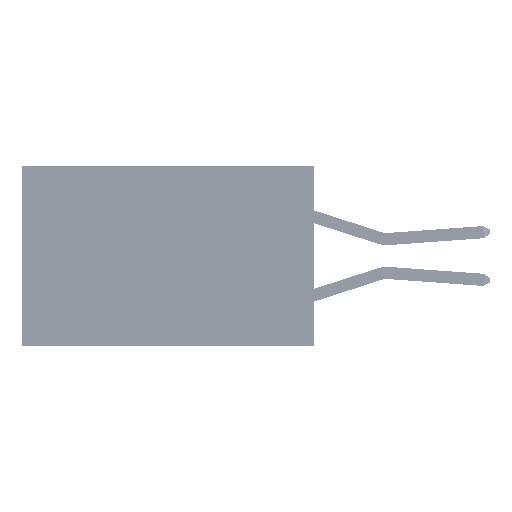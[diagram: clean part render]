
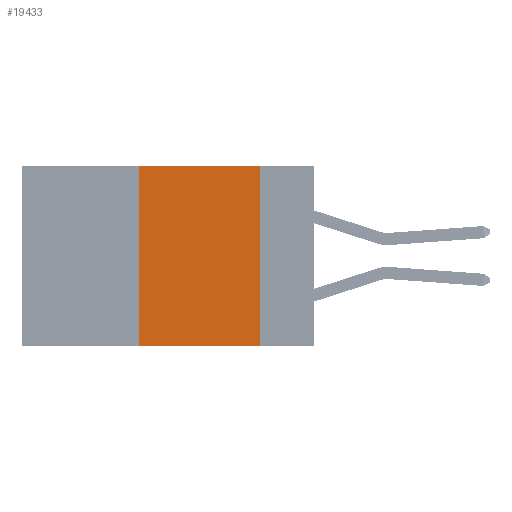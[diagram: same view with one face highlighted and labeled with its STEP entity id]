
A CAD part, left-side view. The second image highlights one B-rep face of the part: STEP entity #19433.
In plain terms, the highlighted planar face has unit normal (-1, 0, 0).
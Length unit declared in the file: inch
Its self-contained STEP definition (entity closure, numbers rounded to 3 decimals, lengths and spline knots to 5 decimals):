
#1965 = CARTESIAN_POINT ( 'NONE',  ( 0., 0.11, -0.37 ) ) ;
#2997 = CARTESIAN_POINT ( 'NONE',  ( 0., 0.36, 0. ) ) ;
#3737 = VERTEX_POINT ( 'NONE', #37068 ) ;
#3966 = ORIENTED_EDGE ( 'NONE', *, *, #29193, .F. ) ;
#3989 = EDGE_LOOP ( 'NONE', ( #7737, #9392, #3966, #5572 ) ) ;
#4426 = EDGE_CURVE ( 'NONE', #3737, #18594, #19802, .T. ) ;
#5292 = AXIS2_PLACEMENT_3D ( 'NONE', #34128, #30416, #40919 ) ;
#5572 = ORIENTED_EDGE ( 'NONE', *, *, #4426, .T. ) ;
#6769 = CARTESIAN_POINT ( 'NONE',  ( 0., 0.11, 0. ) ) ;
#6842 = DIRECTION ( 'NONE',  ( 0., 0., 1. ) ) ;
#7737 = ORIENTED_EDGE ( 'NONE', *, *, #38804, .F. ) ;
#9392 = ORIENTED_EDGE ( 'NONE', *, *, #10692, .F. ) ;
#10190 = VECTOR ( 'NONE', #6842, 39.37008 ) ;
#10692 = EDGE_CURVE ( 'NONE', #22387, #35114, #16682, .T. ) ;
#12783 = PLANE ( 'NONE',  #5292 ) ;
#16682 = LINE ( 'NONE', #24351, #18344 ) ;
#17571 = DIRECTION ( 'NONE',  ( 0., -1., 0. ) ) ;
#18344 = VECTOR ( 'NONE', #41942, 39.37008 ) ;
#18594 = VERTEX_POINT ( 'NONE', #1965 ) ;
#19433 = ADVANCED_FACE ( 'NONE', ( #29479 ), #12783, .F. ) ;
#19802 = LINE ( 'NONE', #20803, #21404 ) ;
#20803 = CARTESIAN_POINT ( 'NONE',  ( 0., 0.6, -0.37 ) ) ;
#21404 = VECTOR ( 'NONE', #17571, 39.37008 ) ;
#22387 = VERTEX_POINT ( 'NONE', #25935 ) ;
#24351 = CARTESIAN_POINT ( 'NONE',  ( 0., 0.6, 0. ) ) ;
#25935 = CARTESIAN_POINT ( 'NONE',  ( 0., 0.36, 0. ) ) ;
#29193 = EDGE_CURVE ( 'NONE', #3737, #22387, #41554, .T. ) ;
#29479 = FACE_OUTER_BOUND ( 'NONE', #3989, .T. ) ;
#30416 = DIRECTION ( 'NONE',  ( 1., 0., 0. ) ) ;
#34128 = CARTESIAN_POINT ( 'NONE',  ( 0., 0.6, 0. ) ) ;
#34395 = DIRECTION ( 'NONE',  ( 0., 0., -1. ) ) ;
#35114 = VERTEX_POINT ( 'NONE', #6769 ) ;
#36094 = VECTOR ( 'NONE', #34395, 39.37008 ) ;
#37068 = CARTESIAN_POINT ( 'NONE',  ( 0., 0.36, -0.37 ) ) ;
#38804 = EDGE_CURVE ( 'NONE', #35114, #18594, #44899, .T. ) ;
#40919 = DIRECTION ( 'NONE',  ( 0., 0., -1. ) ) ;
#41466 = CARTESIAN_POINT ( 'NONE',  ( 0., 0.11, 0. ) ) ;
#41554 = LINE ( 'NONE', #2997, #10190 ) ;
#41942 = DIRECTION ( 'NONE',  ( 0., -1., 0. ) ) ;
#44899 = LINE ( 'NONE', #41466, #36094 ) ;
